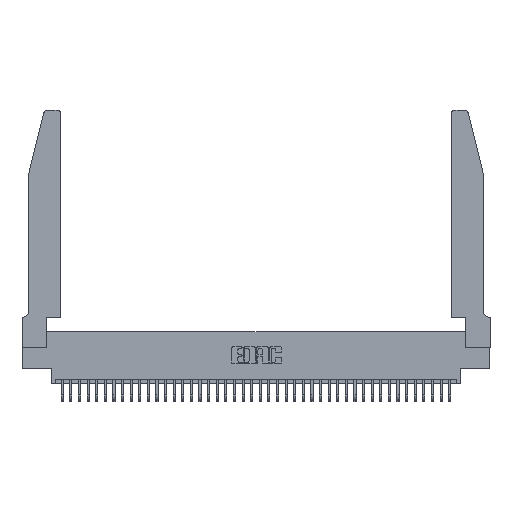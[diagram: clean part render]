
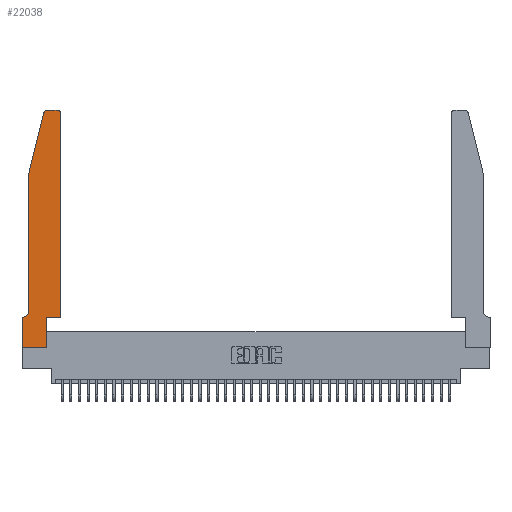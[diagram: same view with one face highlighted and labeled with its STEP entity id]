
A CAD part, top view. The second image highlights one B-rep face of the part: STEP entity #22038.
In plain terms, the highlighted planar face has unit normal (0, 0, 1).
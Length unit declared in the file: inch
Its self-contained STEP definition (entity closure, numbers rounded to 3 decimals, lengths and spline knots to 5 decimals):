
#853 = DIRECTION ( 'NONE',  ( 0., 0., 1. ) ) ;
#934 = LINE ( 'NONE', #38530, #28966 ) ;
#1489 = VECTOR ( 'NONE', #4821, 39.37008 ) ;
#1563 = CARTESIAN_POINT ( 'NONE',  ( 0.2865, 0., 0.37 ) ) ;
#2097 = VERTEX_POINT ( 'NONE', #15720 ) ;
#2618 = LINE ( 'NONE', #5793, #30029 ) ;
#3379 = EDGE_CURVE ( 'NONE', #16744, #5829, #2618, .T. ) ;
#4231 = EDGE_CURVE ( 'NONE', #35685, #25393, #30465, .T. ) ;
#4821 = DIRECTION ( 'NONE',  ( 0., 1., 0. ) ) ;
#5016 = VECTOR ( 'NONE', #18159, 39.37008 ) ;
#5184 = CARTESIAN_POINT ( 'NONE',  ( 0.25487, 2.72718, 0.37 ) ) ;
#5793 = CARTESIAN_POINT ( 'NONE',  ( 0.0755, 0.35, 0.37 ) ) ;
#5829 = VERTEX_POINT ( 'NONE', #35876 ) ;
#5900 = EDGE_LOOP ( 'NONE', ( #35889, #31923, #39640, #7084, #19206, #6098, #25673, #9308, #28474, #36772, #30102, #20838 ) ) ;
#6098 = ORIENTED_EDGE ( 'NONE', *, *, #3379, .T. ) ;
#6184 = CARTESIAN_POINT ( 'NONE',  ( 0.2865, 0.35, 0.37 ) ) ;
#6336 = DIRECTION ( 'NONE',  ( 1., 0., 0. ) ) ;
#6469 = CARTESIAN_POINT ( 'NONE',  ( 0., 0.35, 0.37 ) ) ;
#6749 = CARTESIAN_POINT ( 'NONE',  ( 0.0755, 0.42, 0.37 ) ) ;
#7084 = ORIENTED_EDGE ( 'NONE', *, *, #10148, .T. ) ;
#7177 = CIRCLE ( 'NONE', #39232, 0.03 ) ;
#8679 = CARTESIAN_POINT ( 'NONE',  ( 0.4505, 0.35, 0.37 ) ) ;
#8743 = VERTEX_POINT ( 'NONE', #19673 ) ;
#8949 = CARTESIAN_POINT ( 'NONE',  ( 0.0755, 2., 0.37 ) ) ;
#9020 = EDGE_CURVE ( 'NONE', #26056, #16744, #15042, .T. ) ;
#9308 = ORIENTED_EDGE ( 'NONE', *, *, #24570, .T. ) ;
#10148 = EDGE_CURVE ( 'NONE', #25393, #26056, #33782, .T. ) ;
#10494 = VERTEX_POINT ( 'NONE', #6184 ) ;
#10776 = VECTOR ( 'NONE', #40997, 39.37008 ) ;
#10975 = CARTESIAN_POINT ( 'NONE',  ( 0.4205, 2.72, 0.37 ) ) ;
#12014 = CARTESIAN_POINT ( 'NONE',  ( 0.0055, 0.42, 0.37 ) ) ;
#13473 = FACE_OUTER_BOUND ( 'NONE', #5900, .T. ) ;
#14672 = CARTESIAN_POINT ( 'NONE',  ( 0., 0., 0.37 ) ) ;
#15042 = CIRCLE ( 'NONE', #34798, 0.07 ) ;
#15720 = CARTESIAN_POINT ( 'NONE',  ( 0.4505, 2.72, 0.37 ) ) ;
#15866 = DIRECTION ( 'NONE',  ( 0., 0., -1. ) ) ;
#16744 = VERTEX_POINT ( 'NONE', #20036 ) ;
#16941 = LINE ( 'NONE', #41966, #29637 ) ;
#17803 = CARTESIAN_POINT ( 'NONE',  ( 0.4505, 0.35, 0.37 ) ) ;
#18159 = DIRECTION ( 'NONE',  ( 1., 0., 0. ) ) ;
#18552 = VERTEX_POINT ( 'NONE', #21927 ) ;
#18821 = LINE ( 'NONE', #39263, #1489 ) ;
#18966 = EDGE_CURVE ( 'NONE', #38446, #10494, #18821, .T. ) ;
#19055 = DIRECTION ( 'NONE',  ( 1., 0., 0. ) ) ;
#19206 = ORIENTED_EDGE ( 'NONE', *, *, #9020, .T. ) ;
#19577 = CIRCLE ( 'NONE', #39918, 0.03 ) ;
#19673 = CARTESIAN_POINT ( 'NONE',  ( 0.4205, 2.75, 0.37 ) ) ;
#20036 = CARTESIAN_POINT ( 'NONE',  ( 0.0055, 0.35, 0.37 ) ) ;
#20551 = DIRECTION ( 'NONE',  ( 0., -1., 0. ) ) ;
#20838 = ORIENTED_EDGE ( 'NONE', *, *, #22840, .T. ) ;
#21349 = DIRECTION ( 'NONE',  ( -1., 0., 0. ) ) ;
#21927 = CARTESIAN_POINT ( 'NONE',  ( 0.284, 2.75, 0.37 ) ) ;
#22038 = ADVANCED_FACE ( 'NONE', ( #13473 ), #25854, .T. ) ;
#22064 = CARTESIAN_POINT ( 'NONE',  ( 0.0755, 2., 0.37 ) ) ;
#22542 = DIRECTION ( 'NONE',  ( 0., 0., 1. ) ) ;
#22840 = EDGE_CURVE ( 'NONE', #2097, #8743, #7177, .T. ) ;
#24189 = EDGE_CURVE ( 'NONE', #10494, #31725, #934, .T. ) ;
#24570 = EDGE_CURVE ( 'NONE', #34357, #38446, #34002, .T. ) ;
#25088 = LINE ( 'NONE', #14672, #26556 ) ;
#25256 = CARTESIAN_POINT ( 'NONE',  ( 0.284, 2.72, 0.37 ) ) ;
#25333 = DIRECTION ( 'NONE',  ( -0.239, -0.971, 0. ) ) ;
#25335 = DIRECTION ( 'NONE',  ( 0., -1., 0. ) ) ;
#25393 = VERTEX_POINT ( 'NONE', #41670 ) ;
#25426 = VECTOR ( 'NONE', #25333, 39.37008 ) ;
#25673 = ORIENTED_EDGE ( 'NONE', *, *, #35942, .T. ) ;
#25854 = PLANE ( 'NONE',  #38131 ) ;
#26056 = VERTEX_POINT ( 'NONE', #6749 ) ;
#26556 = VECTOR ( 'NONE', #20551, 39.37008 ) ;
#26637 = VECTOR ( 'NONE', #25335, 39.37008 ) ;
#27884 = CARTESIAN_POINT ( 'NONE',  ( 0., 0., 0.37 ) ) ;
#28048 = EDGE_CURVE ( 'NONE', #18552, #35685, #19577, .T. ) ;
#28474 = ORIENTED_EDGE ( 'NONE', *, *, #18966, .T. ) ;
#28622 = EDGE_CURVE ( 'NONE', #8743, #18552, #16941, .T. ) ;
#28966 = VECTOR ( 'NONE', #19055, 39.37008 ) ;
#29236 = DIRECTION ( 'NONE',  ( 0., 0., 1. ) ) ;
#29637 = VECTOR ( 'NONE', #32118, 39.37008 ) ;
#30029 = VECTOR ( 'NONE', #21349, 39.37008 ) ;
#30102 = ORIENTED_EDGE ( 'NONE', *, *, #36112, .T. ) ;
#30465 = LINE ( 'NONE', #8949, #25426 ) ;
#31725 = VERTEX_POINT ( 'NONE', #17803 ) ;
#31923 = ORIENTED_EDGE ( 'NONE', *, *, #28048, .T. ) ;
#32118 = DIRECTION ( 'NONE',  ( -1., 0., 0. ) ) ;
#33782 = LINE ( 'NONE', #22064, #26637 ) ;
#33998 = DIRECTION ( 'NONE',  ( 1., 0., 0. ) ) ;
#34002 = LINE ( 'NONE', #37198, #5016 ) ;
#34148 = LINE ( 'NONE', #8679, #10776 ) ;
#34357 = VERTEX_POINT ( 'NONE', #27884 ) ;
#34798 = AXIS2_PLACEMENT_3D ( 'NONE', #12014, #15866, #41893 ) ;
#35043 = DIRECTION ( 'NONE',  ( 1., 0., 0. ) ) ;
#35685 = VERTEX_POINT ( 'NONE', #5184 ) ;
#35876 = CARTESIAN_POINT ( 'NONE',  ( 0., 0.35, 0.37 ) ) ;
#35889 = ORIENTED_EDGE ( 'NONE', *, *, #28622, .T. ) ;
#35942 = EDGE_CURVE ( 'NONE', #5829, #34357, #25088, .T. ) ;
#36112 = EDGE_CURVE ( 'NONE', #31725, #2097, #34148, .T. ) ;
#36772 = ORIENTED_EDGE ( 'NONE', *, *, #24189, .T. ) ;
#37198 = CARTESIAN_POINT ( 'NONE',  ( 0., 0., 0.37 ) ) ;
#38131 = AXIS2_PLACEMENT_3D ( 'NONE', #6469, #29236, #6336 ) ;
#38446 = VERTEX_POINT ( 'NONE', #1563 ) ;
#38530 = CARTESIAN_POINT ( 'NONE',  ( 0.4505, 0.35, 0.37 ) ) ;
#39232 = AXIS2_PLACEMENT_3D ( 'NONE', #10975, #853, #33998 ) ;
#39263 = CARTESIAN_POINT ( 'NONE',  ( 0.2865, 0.35, 0.37 ) ) ;
#39640 = ORIENTED_EDGE ( 'NONE', *, *, #4231, .T. ) ;
#39918 = AXIS2_PLACEMENT_3D ( 'NONE', #25256, #22542, #35043 ) ;
#40997 = DIRECTION ( 'NONE',  ( 0., 1., 0. ) ) ;
#41670 = CARTESIAN_POINT ( 'NONE',  ( 0.0755, 2., 0.37 ) ) ;
#41893 = DIRECTION ( 'NONE',  ( -1., 0., 0. ) ) ;
#41966 = CARTESIAN_POINT ( 'NONE',  ( 0.2605, 2.75, 0.37 ) ) ;
